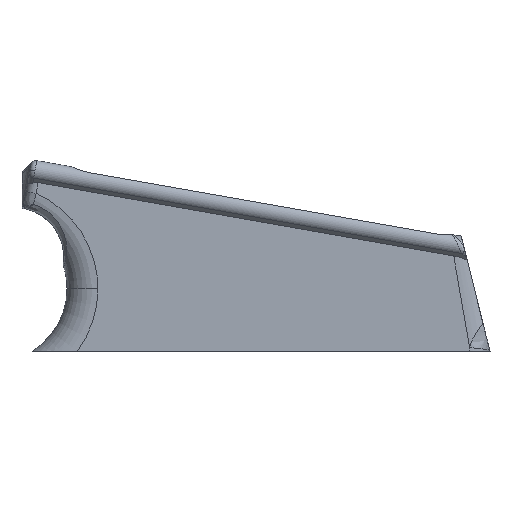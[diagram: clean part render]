
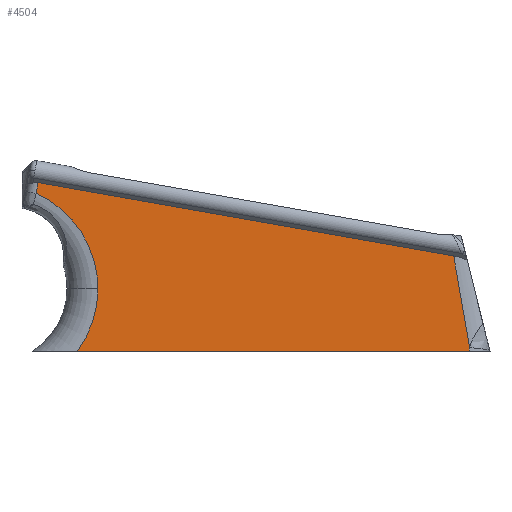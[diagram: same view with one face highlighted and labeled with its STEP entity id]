
A CAD part, front view. The second image highlights one B-rep face of the part: STEP entity #4504.
In plain terms, the highlighted planar face has unit normal (0, -1, 0).
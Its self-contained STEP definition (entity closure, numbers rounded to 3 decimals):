
#31 = AXIS2_PLACEMENT_3D ( 'NONE', #7487, #2402, #4344 ) ;
#189 = CARTESIAN_POINT ( 'NONE',  ( 85.32, -76.726, 19.243 ) ) ;
#205 = EDGE_CURVE ( 'NONE', #3238, #5663, #6139, .T. ) ;
#257 = CARTESIAN_POINT ( 'NONE',  ( 91.879, -76.726, 12.003 ) ) ;
#289 = CARTESIAN_POINT ( 'NONE',  ( 169.1, -76.726, -12.792 ) ) ;
#295 = CARTESIAN_POINT ( 'NONE',  ( 92.9, -76.726, -13.516 ) ) ;
#604 = CARTESIAN_POINT ( 'NONE',  ( 76.653, -76.726, -1.367 ) ) ;
#631 = ORIENTED_EDGE ( 'NONE', *, *, #3379, .T. ) ;
#655 = DIRECTION ( 'NONE',  ( 1., 0., 0. ) ) ;
#811 = VECTOR ( 'NONE', #3725, 1000. ) ;
#882 = CARTESIAN_POINT ( 'NONE',  ( 91.911, -76.726, 12.003 ) ) ;
#1147 = EDGE_CURVE ( 'NONE', #3324, #4377, #5807, .T. ) ;
#1259 = DIRECTION ( 'NONE',  ( -0.008, 0., -1. ) ) ;
#1282 = ORIENTED_EDGE ( 'NONE', *, *, #3128, .T. ) ;
#1310 = ORIENTED_EDGE ( 'NONE', *, *, #205, .T. ) ;
#1375 = DIRECTION ( 'NONE',  ( 0., 1., 0. ) ) ;
#1423 = VECTOR ( 'NONE', #1739, 1000. ) ;
#1469 = AXIS2_PLACEMENT_3D ( 'NONE', #4877, #7937, #3119 ) ;
#1590 = ORIENTED_EDGE ( 'NONE', *, *, #6245, .T. ) ;
#1609 = VERTEX_POINT ( 'NONE', #5295 ) ;
#1650 = CARTESIAN_POINT ( 'NONE',  ( 169.046, -76.726, -13.516 ) ) ;
#1726 = CARTESIAN_POINT ( 'NONE',  ( 85.32, -76.726, 19.243 ) ) ;
#1739 = DIRECTION ( 'NONE',  ( 1., 0., -0.008 ) ) ;
#1743 = CARTESIAN_POINT ( 'NONE',  ( 76.653, -76.726, -1.367 ) ) ;
#1770 = DIRECTION ( 'NONE',  ( -0.174, 0., -0.985 ) ) ;
#1864 = VERTEX_POINT ( 'NONE', #5633 ) ;
#1895 = CARTESIAN_POINT ( 'NONE',  ( 91.879, -76.726, 12.04 ) ) ;
#1988 = DIRECTION ( 'NONE',  ( -0.171, 0., 0.985 ) ) ;
#1996 = CARTESIAN_POINT ( 'NONE',  ( 145.598, -76.726, -13.516 ) ) ;
#2016 = VECTOR ( 'NONE', #1988, 1000. ) ;
#2110 = CIRCLE ( 'NONE', #6467, 20.288 ) ;
#2379 = EDGE_CURVE ( 'NONE', #3703, #1609, #3236, .T. ) ;
#2402 = DIRECTION ( 'NONE',  ( 0., 1., 0. ) ) ;
#2477 = LINE ( 'NONE', #3125, #811 ) ;
#2513 = LINE ( 'NONE', #4236, #3410 ) ;
#3113 = LINE ( 'NONE', #1726, #3894 ) ;
#3119 = DIRECTION ( 'NONE',  ( 0., 0., 1. ) ) ;
#3124 = CARTESIAN_POINT ( 'NONE',  ( 146.013, -76.726, 11.546 ) ) ;
#3125 = CARTESIAN_POINT ( 'NONE',  ( 151.241, -76.726, 7.619 ) ) ;
#3128 = EDGE_CURVE ( 'NONE', #5663, #3337, #6766, .T. ) ;
#3236 = LINE ( 'NONE', #289, #2016 ) ;
#3238 = VERTEX_POINT ( 'NONE', #257 ) ;
#3324 = VERTEX_POINT ( 'NONE', #295 ) ;
#3337 = VERTEX_POINT ( 'NONE', #5812 ) ;
#3379 = EDGE_CURVE ( 'NONE', #7164, #3238, #2513, .T. ) ;
#3410 = VECTOR ( 'NONE', #1259, 1000. ) ;
#3630 = PLANE ( 'NONE',  #1469 ) ;
#3703 = VERTEX_POINT ( 'NONE', #7925 ) ;
#3725 = DIRECTION ( 'NONE',  ( 0.985, 0., -0.174 ) ) ;
#3823 = EDGE_CURVE ( 'NONE', #3337, #3324, #2110, .T. ) ;
#3894 = VECTOR ( 'NONE', #1770, 1000. ) ;
#3922 = DIRECTION ( 'NONE',  ( 1., 0., 0. ) ) ;
#4199 = FACE_OUTER_BOUND ( 'NONE', #4355, .T. ) ;
#4207 = DIRECTION ( 'NONE',  ( 1., 0., 0. ) ) ;
#4236 = CARTESIAN_POINT ( 'NONE',  ( 91.464, -76.726, -37.113 ) ) ;
#4317 = VERTEX_POINT ( 'NONE', #189 ) ;
#4344 = DIRECTION ( 'NONE',  ( 1., 0., 0. ) ) ;
#4355 = EDGE_LOOP ( 'NONE', ( #1282, #4751, #6941, #7238, #4385, #6891, #1590, #6074, #631, #1310 ) ) ;
#4377 = VERTEX_POINT ( 'NONE', #1650 ) ;
#4385 = ORIENTED_EDGE ( 'NONE', *, *, #2379, .T. ) ;
#4439 = AXIS2_PLACEMENT_3D ( 'NONE', #604, #7362, #7451 ) ;
#4504 = ADVANCED_FACE ( 'NONE', ( #4199 ), #3630, .F. ) ;
#4659 = EDGE_CURVE ( 'NONE', #1864, #7164, #4805, .T. ) ;
#4751 = ORIENTED_EDGE ( 'NONE', *, *, #3823, .T. ) ;
#4805 = CIRCLE ( 'NONE', #4439, 20.288 ) ;
#4877 = CARTESIAN_POINT ( 'NONE',  ( 145.598, -76.726, -37.57 ) ) ;
#4915 = CARTESIAN_POINT ( 'NONE',  ( 76.653, -76.726, -1.367 ) ) ;
#5295 = CARTESIAN_POINT ( 'NONE',  ( 166.002, -76.726, 5.016 ) ) ;
#5633 = CARTESIAN_POINT ( 'NONE',  ( 84.95, -76.726, 17.146 ) ) ;
#5663 = VERTEX_POINT ( 'NONE', #882 ) ;
#5807 = LINE ( 'NONE', #1996, #7197 ) ;
#5812 = CARTESIAN_POINT ( 'NONE',  ( 96.94, -76.726, -1.367 ) ) ;
#6023 = EDGE_CURVE ( 'NONE', #4317, #1609, #2477, .T. ) ;
#6074 = ORIENTED_EDGE ( 'NONE', *, *, #4659, .T. ) ;
#6139 = LINE ( 'NONE', #3124, #1423 ) ;
#6245 = EDGE_CURVE ( 'NONE', #4317, #1864, #3113, .T. ) ;
#6467 = AXIS2_PLACEMENT_3D ( 'NONE', #4915, #1375, #655 ) ;
#6623 = AXIS2_PLACEMENT_3D ( 'NONE', #1743, #6739, #4207 ) ;
#6739 = DIRECTION ( 'NONE',  ( 0., 1., 0. ) ) ;
#6766 = CIRCLE ( 'NONE', #6623, 20.288 ) ;
#6864 = EDGE_CURVE ( 'NONE', #4377, #3703, #6974, .T. ) ;
#6891 = ORIENTED_EDGE ( 'NONE', *, *, #6023, .F. ) ;
#6941 = ORIENTED_EDGE ( 'NONE', *, *, #1147, .T. ) ;
#6974 = CIRCLE ( 'NONE', #31, 14. ) ;
#7164 = VERTEX_POINT ( 'NONE', #1895 ) ;
#7197 = VECTOR ( 'NONE', #3922, 1000. ) ;
#7238 = ORIENTED_EDGE ( 'NONE', *, *, #6864, .T. ) ;
#7362 = DIRECTION ( 'NONE',  ( 0., 1., 0. ) ) ;
#7451 = DIRECTION ( 'NONE',  ( 1., 0., 0. ) ) ;
#7487 = CARTESIAN_POINT ( 'NONE',  ( 183.03, -76.726, -14.191 ) ) ;
#7925 = CARTESIAN_POINT ( 'NONE',  ( 169.1, -76.726, -12.792 ) ) ;
#7937 = DIRECTION ( 'NONE',  ( 0., 1., 0. ) ) ;
